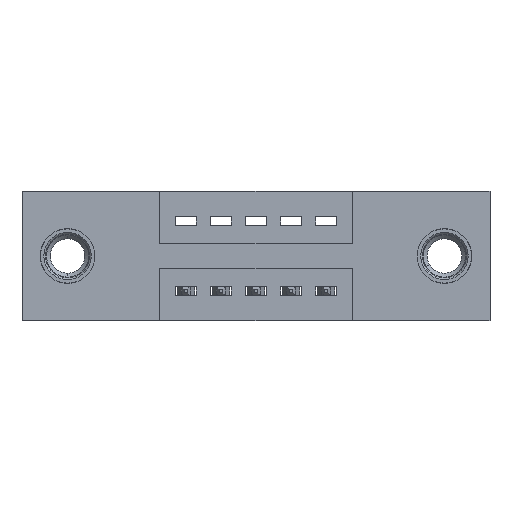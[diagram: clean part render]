
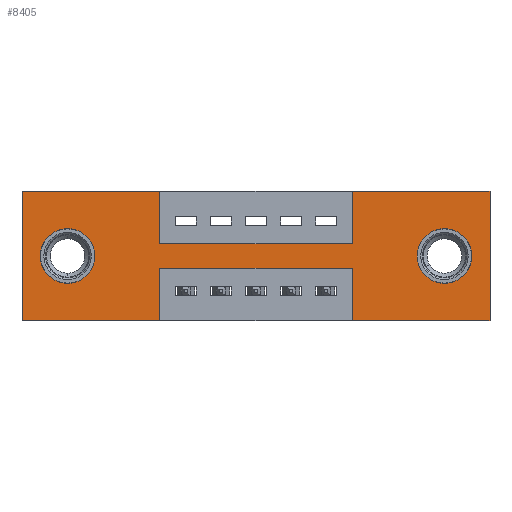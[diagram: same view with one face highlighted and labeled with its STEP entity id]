
A CAD part, front view. The second image highlights one B-rep face of the part: STEP entity #8405.
In plain terms, the highlighted planar face has unit normal (0, -1, 0).
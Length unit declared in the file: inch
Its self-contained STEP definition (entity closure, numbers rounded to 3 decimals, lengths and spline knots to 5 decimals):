
#2 = DIRECTION ( 'NONE',  ( -1., 0., 0. ) ) ;
#46 = DIRECTION ( 'NONE',  ( 0., 0., 1. ) ) ;
#88 = LINE ( 'NONE', #5390, #8413 ) ;
#106 = VERTEX_POINT ( 'NONE', #8128 ) ;
#174 = DIRECTION ( 'NONE',  ( 0., 0., -1. ) ) ;
#175 = CARTESIAN_POINT ( 'NONE',  ( 0.3925, 0., -0.22 ) ) ;
#211 = LINE ( 'NONE', #501, #2269 ) ;
#218 = ORIENTED_EDGE ( 'NONE', *, *, #7877, .F. ) ;
#238 = LINE ( 'NONE', #6792, #4900 ) ;
#273 = CARTESIAN_POINT ( 'NONE',  ( 0., 0., 0. ) ) ;
#293 = EDGE_CURVE ( 'NONE', #7679, #3046, #4510, .T. ) ;
#500 = DIRECTION ( 'NONE',  ( 1., 0., 0. ) ) ;
#501 = CARTESIAN_POINT ( 'NONE',  ( 0.9425, 0., 0. ) ) ;
#527 = CARTESIAN_POINT ( 'NONE',  ( 0.9425, 0., 0. ) ) ;
#575 = VECTOR ( 'NONE', #2, 39.37008 ) ;
#658 = VERTEX_POINT ( 'NONE', #8798 ) ;
#666 = AXIS2_PLACEMENT_3D ( 'NONE', #8708, #4348, #9429 ) ;
#728 = CARTESIAN_POINT ( 'NONE',  ( 0.13, 0., -0.263 ) ) ;
#847 = LINE ( 'NONE', #906, #575 ) ;
#872 = CARTESIAN_POINT ( 'NONE',  ( 0.3925, 0., -0.15 ) ) ;
#906 = CARTESIAN_POINT ( 'NONE',  ( 0., 0., -0.37 ) ) ;
#1055 = ORIENTED_EDGE ( 'NONE', *, *, #6409, .F. ) ;
#1067 = VERTEX_POINT ( 'NONE', #2313 ) ;
#1076 = CIRCLE ( 'NONE', #8700, 0.078 ) ;
#1173 = DIRECTION ( 'NONE',  ( 0., 0., 1. ) ) ;
#1193 = VERTEX_POINT ( 'NONE', #175 ) ;
#1287 = CARTESIAN_POINT ( 'NONE',  ( 1.335, 0., 0. ) ) ;
#1352 = VECTOR ( 'NONE', #3560, 39.37008 ) ;
#1631 = LINE ( 'NONE', #8703, #1352 ) ;
#1704 = LINE ( 'NONE', #5809, #3658 ) ;
#1720 = VERTEX_POINT ( 'NONE', #6031 ) ;
#1876 = ORIENTED_EDGE ( 'NONE', *, *, #5741, .F. ) ;
#1893 = DIRECTION ( 'NONE',  ( 1., 0., 0. ) ) ;
#1954 = ORIENTED_EDGE ( 'NONE', *, *, #7026, .F. ) ;
#2142 = CIRCLE ( 'NONE', #8606, 0.078 ) ;
#2180 = DIRECTION ( 'NONE',  ( -1., 0., 0. ) ) ;
#2259 = VECTOR ( 'NONE', #174, 39.37008 ) ;
#2261 = ORIENTED_EDGE ( 'NONE', *, *, #6851, .T. ) ;
#2269 = VECTOR ( 'NONE', #4662, 39.37008 ) ;
#2313 = CARTESIAN_POINT ( 'NONE',  ( 0.9425, 0., -0.37 ) ) ;
#2555 = LINE ( 'NONE', #1287, #6637 ) ;
#2603 = EDGE_LOOP ( 'NONE', ( #2261, #4002 ) ) ;
#2611 = FACE_BOUND ( 'NONE', #3391, .T. ) ;
#2666 = VERTEX_POINT ( 'NONE', #5509 ) ;
#2713 = VERTEX_POINT ( 'NONE', #728 ) ;
#2882 = FACE_BOUND ( 'NONE', #2603, .T. ) ;
#3046 = VERTEX_POINT ( 'NONE', #4461 ) ;
#3297 = CARTESIAN_POINT ( 'NONE',  ( 1.205, 0., -0.263 ) ) ;
#3298 = ORIENTED_EDGE ( 'NONE', *, *, #3636, .F. ) ;
#3391 = EDGE_LOOP ( 'NONE', ( #4620, #4396 ) ) ;
#3404 = VECTOR ( 'NONE', #1173, 39.37008 ) ;
#3460 = CARTESIAN_POINT ( 'NONE',  ( 1.205, 0., -0.185 ) ) ;
#3560 = DIRECTION ( 'NONE',  ( 0., 0., -1. ) ) ;
#3636 = EDGE_CURVE ( 'NONE', #1193, #2666, #1631, .T. ) ;
#3658 = VECTOR ( 'NONE', #1893, 39.37008 ) ;
#3686 = DIRECTION ( 'NONE',  ( 0., 1., 0. ) ) ;
#3774 = EDGE_CURVE ( 'NONE', #7395, #1193, #8317, .T. ) ;
#3781 = VERTEX_POINT ( 'NONE', #6003 ) ;
#3867 = VERTEX_POINT ( 'NONE', #6837 ) ;
#3886 = CARTESIAN_POINT ( 'NONE',  ( 0.3925, 0., -0.15 ) ) ;
#4002 = ORIENTED_EDGE ( 'NONE', *, *, #6095, .T. ) ;
#4071 = VERTEX_POINT ( 'NONE', #3297 ) ;
#4249 = DIRECTION ( 'NONE',  ( 0., 0., -1. ) ) ;
#4261 = CARTESIAN_POINT ( 'NONE',  ( 0., 0., -0.37 ) ) ;
#4348 = DIRECTION ( 'NONE',  ( 0., 1., 0. ) ) ;
#4359 = CIRCLE ( 'NONE', #666, 0.078 ) ;
#4396 = ORIENTED_EDGE ( 'NONE', *, *, #7322, .T. ) ;
#4461 = CARTESIAN_POINT ( 'NONE',  ( 1.335, 0., 0. ) ) ;
#4465 = CARTESIAN_POINT ( 'NONE',  ( 0., 0., 0. ) ) ;
#4473 = EDGE_CURVE ( 'NONE', #2666, #658, #238, .T. ) ;
#4486 = CARTESIAN_POINT ( 'NONE',  ( 0.3925, 0., -0.22 ) ) ;
#4510 = LINE ( 'NONE', #4465, #9796 ) ;
#4620 = ORIENTED_EDGE ( 'NONE', *, *, #9090, .T. ) ;
#4662 = DIRECTION ( 'NONE',  ( 0., 0., 1. ) ) ;
#4846 = AXIS2_PLACEMENT_3D ( 'NONE', #3460, #8612, #4249 ) ;
#4900 = VECTOR ( 'NONE', #2180, 39.37008 ) ;
#4998 = DIRECTION ( 'NONE',  ( 0., 1., 0. ) ) ;
#5015 = DIRECTION ( 'NONE',  ( 0., 0., -1. ) ) ;
#5042 = CARTESIAN_POINT ( 'NONE',  ( 0.9425, 0., -0.22 ) ) ;
#5114 = AXIS2_PLACEMENT_3D ( 'NONE', #4261, #9343, #5015 ) ;
#5390 = CARTESIAN_POINT ( 'NONE',  ( 0.9425, 0., -0.37 ) ) ;
#5422 = VECTOR ( 'NONE', #500, 39.37008 ) ;
#5459 = ORIENTED_EDGE ( 'NONE', *, *, #8723, .F. ) ;
#5509 = CARTESIAN_POINT ( 'NONE',  ( 0.3925, 0., -0.37 ) ) ;
#5741 = EDGE_CURVE ( 'NONE', #3046, #6801, #2555, .T. ) ;
#5809 = CARTESIAN_POINT ( 'NONE',  ( 0., 0., 0. ) ) ;
#5860 = CARTESIAN_POINT ( 'NONE',  ( 0.3925, 0., 0. ) ) ;
#6003 = CARTESIAN_POINT ( 'NONE',  ( 0.9425, 0., -0.15 ) ) ;
#6031 = CARTESIAN_POINT ( 'NONE',  ( 0.13, 0., -0.107 ) ) ;
#6048 = DIRECTION ( 'NONE',  ( 0., 0., -1. ) ) ;
#6095 = EDGE_CURVE ( 'NONE', #2713, #1720, #1076, .T. ) ;
#6391 = VECTOR ( 'NONE', #7441, 39.37008 ) ;
#6409 = EDGE_CURVE ( 'NONE', #1067, #7395, #88, .T. ) ;
#6637 = VECTOR ( 'NONE', #6048, 39.37008 ) ;
#6686 = FACE_OUTER_BOUND ( 'NONE', #8387, .T. ) ;
#6786 = VERTEX_POINT ( 'NONE', #5860 ) ;
#6792 = CARTESIAN_POINT ( 'NONE',  ( 0., 0., -0.37 ) ) ;
#6801 = VERTEX_POINT ( 'NONE', #8036 ) ;
#6837 = CARTESIAN_POINT ( 'NONE',  ( 1.205, 0., -0.107 ) ) ;
#6851 = EDGE_CURVE ( 'NONE', #1720, #2713, #2142, .T. ) ;
#7026 = EDGE_CURVE ( 'NONE', #3781, #7679, #211, .T. ) ;
#7285 = CIRCLE ( 'NONE', #4846, 0.078 ) ;
#7322 = EDGE_CURVE ( 'NONE', #4071, #3867, #7285, .T. ) ;
#7327 = DIRECTION ( 'NONE',  ( 1., 0., 0. ) ) ;
#7395 = VERTEX_POINT ( 'NONE', #5042 ) ;
#7415 = ORIENTED_EDGE ( 'NONE', *, *, #7433, .F. ) ;
#7433 = EDGE_CURVE ( 'NONE', #6786, #7792, #8288, .T. ) ;
#7441 = DIRECTION ( 'NONE',  ( -1., 0., 0. ) ) ;
#7505 = EDGE_CURVE ( 'NONE', #658, #106, #9271, .T. ) ;
#7679 = VERTEX_POINT ( 'NONE', #527 ) ;
#7792 = VERTEX_POINT ( 'NONE', #872 ) ;
#7877 = EDGE_CURVE ( 'NONE', #106, #6786, #1704, .T. ) ;
#7904 = PLANE ( 'NONE',  #5114 ) ;
#8035 = ORIENTED_EDGE ( 'NONE', *, *, #7505, .F. ) ;
#8036 = CARTESIAN_POINT ( 'NONE',  ( 1.335, 0., -0.37 ) ) ;
#8104 = CARTESIAN_POINT ( 'NONE',  ( 0.13, 0., -0.185 ) ) ;
#8128 = CARTESIAN_POINT ( 'NONE',  ( 0., 0., 0. ) ) ;
#8288 = LINE ( 'NONE', #9430, #2259 ) ;
#8292 = ORIENTED_EDGE ( 'NONE', *, *, #293, .F. ) ;
#8317 = LINE ( 'NONE', #4486, #6391 ) ;
#8387 = EDGE_LOOP ( 'NONE', ( #3298, #9814, #1055, #8502, #1876, #8292, #1954, #5459, #7415, #218, #8035, #9257 ) ) ;
#8405 = ADVANCED_FACE ( 'NONE', ( #2611, #2882, #6686 ), #7904, .T. ) ;
#8413 = VECTOR ( 'NONE', #9687, 39.37008 ) ;
#8502 = ORIENTED_EDGE ( 'NONE', *, *, #9602, .F. ) ;
#8606 = AXIS2_PLACEMENT_3D ( 'NONE', #8104, #3686, #8812 ) ;
#8612 = DIRECTION ( 'NONE',  ( 0., 1., 0. ) ) ;
#8700 = AXIS2_PLACEMENT_3D ( 'NONE', #9324, #4998, #46 ) ;
#8703 = CARTESIAN_POINT ( 'NONE',  ( 0.3925, 0., -0.37 ) ) ;
#8708 = CARTESIAN_POINT ( 'NONE',  ( 1.205, 0., -0.185 ) ) ;
#8723 = EDGE_CURVE ( 'NONE', #7792, #3781, #9245, .T. ) ;
#8798 = CARTESIAN_POINT ( 'NONE',  ( 0., 0., -0.37 ) ) ;
#8812 = DIRECTION ( 'NONE',  ( 0., 0., 1. ) ) ;
#9090 = EDGE_CURVE ( 'NONE', #3867, #4071, #4359, .T. ) ;
#9245 = LINE ( 'NONE', #3886, #5422 ) ;
#9257 = ORIENTED_EDGE ( 'NONE', *, *, #4473, .F. ) ;
#9271 = LINE ( 'NONE', #273, #3404 ) ;
#9324 = CARTESIAN_POINT ( 'NONE',  ( 0.13, 0., -0.185 ) ) ;
#9343 = DIRECTION ( 'NONE',  ( 0., -1., 0. ) ) ;
#9429 = DIRECTION ( 'NONE',  ( 0., 0., -1. ) ) ;
#9430 = CARTESIAN_POINT ( 'NONE',  ( 0.3925, 0., 0. ) ) ;
#9602 = EDGE_CURVE ( 'NONE', #6801, #1067, #847, .T. ) ;
#9687 = DIRECTION ( 'NONE',  ( 0., 0., 1. ) ) ;
#9796 = VECTOR ( 'NONE', #7327, 39.37008 ) ;
#9814 = ORIENTED_EDGE ( 'NONE', *, *, #3774, .F. ) ;
